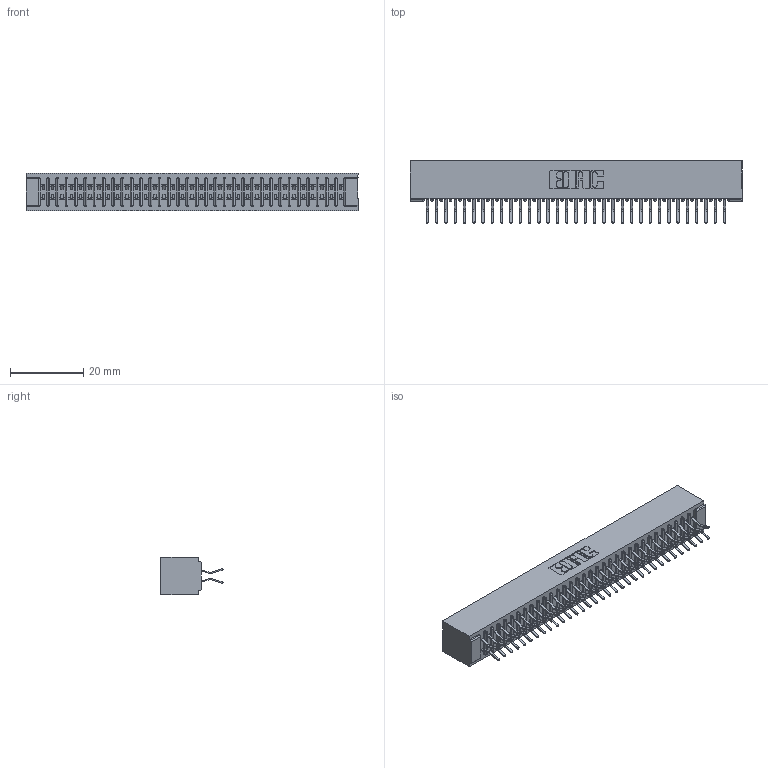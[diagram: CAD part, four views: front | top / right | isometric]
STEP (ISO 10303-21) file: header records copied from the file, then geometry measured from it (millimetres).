
FILE_DESCRIPTION (( 'STEP AP203' ), '1' );
FILE_NAME ('391-066-556-201.STEP', '2018-08-09T13:34:54', ( '' ), ( '' ), 'SwSTEP 2.0', 'SolidWorks 2016', '' );
FILE_SCHEMA (( 'CONFIG_CONTROL_DESIGN' ));
Length unit declared in the file: inch
Products named in the file (3): 341-292-001_341-292-156; 391-066-556-201; 341 Part_No Mounting Lugs
Assembly tree (67 placements, depth 2):
  391-066-556-201
    341 Part_No Mounting Lugs
    341-292-001_341-292-156  x66
Bounding box: 90.81 x 17.07 x 10.16 mm (x, y, z)
Volume: 6954.4 mm3; surface area: 12880.9 mm2
Topology: 67 solids, 67 shells, 4728 faces, 13723 edges, 8902 vertices
Faces by surface type: plane 2704, cylinder 1892, sphere 68, torus 64
Entity records: 40998 total; most frequent: CARTESIAN_POINT 6815, ORIENTED_EDGE 6770, DIRECTION 6623, EDGE_CURVE 3385, LINE 2723, VECTOR 2723, VERTEX_POINT 2142, AXIS2_PLACEMENT_3D 1950
